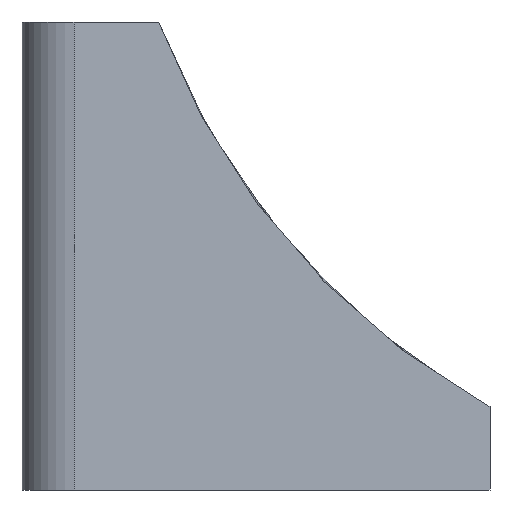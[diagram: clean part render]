
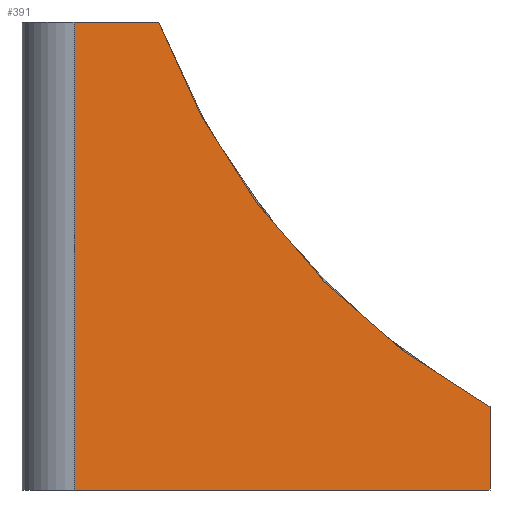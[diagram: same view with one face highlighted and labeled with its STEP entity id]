
A CAD part, left-side view. The second image highlights one B-rep face of the part: STEP entity #391.
In plain terms, the highlighted planar face has unit normal (-0.992, -0.124, 0).
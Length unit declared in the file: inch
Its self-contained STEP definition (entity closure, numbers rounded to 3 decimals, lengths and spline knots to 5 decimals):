
#25=PLANE('',#438);
#35=ELLIPSE('',#434,3.52724,3.5);
#41=FACE_OUTER_BOUND('',#62,.T.);
#62=EDGE_LOOP('',(#288,#289,#290,#291,#292));
#95=LINE('',#633,#127);
#100=LINE('',#643,#132);
#101=LINE('',#645,#133);
#102=LINE('',#646,#134);
#127=VECTOR('',#504,0.3937);
#132=VECTOR('',#513,0.3937);
#133=VECTOR('',#514,0.3937);
#134=VECTOR('',#515,0.3937);
#179=VERTEX_POINT('',#618);
#180=VERTEX_POINT('',#620);
#184=VERTEX_POINT('',#632);
#187=VERTEX_POINT('',#642);
#188=VERTEX_POINT('',#644);
#217=EDGE_CURVE('',#180,#179,#35,.T.);
#223=EDGE_CURVE('',#184,#180,#95,.T.);
#228=EDGE_CURVE('',#187,#179,#100,.T.);
#229=EDGE_CURVE('',#188,#187,#101,.T.);
#230=EDGE_CURVE('',#188,#184,#102,.T.);
#288=ORIENTED_EDGE('',*,*,#217,.T.);
#289=ORIENTED_EDGE('',*,*,#228,.F.);
#290=ORIENTED_EDGE('',*,*,#229,.F.);
#291=ORIENTED_EDGE('',*,*,#230,.T.);
#292=ORIENTED_EDGE('',*,*,#223,.T.);
#391=ADVANCED_FACE('',(#41),#25,.T.);
#434=AXIS2_PLACEMENT_3D('',#621,#493,#494);
#438=AXIS2_PLACEMENT_3D('',#641,#511,#512);
#493=DIRECTION('center_axis',(0.992,0.124,0.));
#494=DIRECTION('ref_axis',(-0.124,0.992,0.));
#504=DIRECTION('',(0.,0.,1.));
#511=DIRECTION('center_axis',(-0.992,-0.124,0.));
#512=DIRECTION('ref_axis',(0.124,-0.992,0.));
#513=DIRECTION('',(0.124,-0.992,0.));
#514=DIRECTION('',(0.,0.,1.));
#515=DIRECTION('',(0.124,-0.992,0.));
#618=CARTESIAN_POINT('',(-0.19904,1.59233,2.25));
#620=CARTESIAN_POINT('',(0.,0.,0.4));
#621=CARTESIAN_POINT('Origin',(0.21126,-1.69004,3.46492));
#632=CARTESIAN_POINT('',(0.,0.,0.));
#633=CARTESIAN_POINT('',(0.,0.,0.));
#641=CARTESIAN_POINT('Origin',(-0.25,2.,0.));
#642=CARTESIAN_POINT('',(-0.25,2.,2.25));
#643=CARTESIAN_POINT('',(-0.25,2.,2.25));
#644=CARTESIAN_POINT('',(-0.25,2.,0.));
#645=CARTESIAN_POINT('',(-0.25,2.,0.));
#646=CARTESIAN_POINT('',(-0.25,2.,0.));
